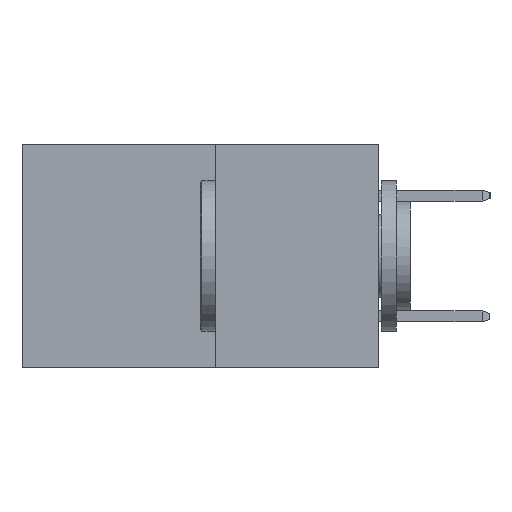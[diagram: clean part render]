
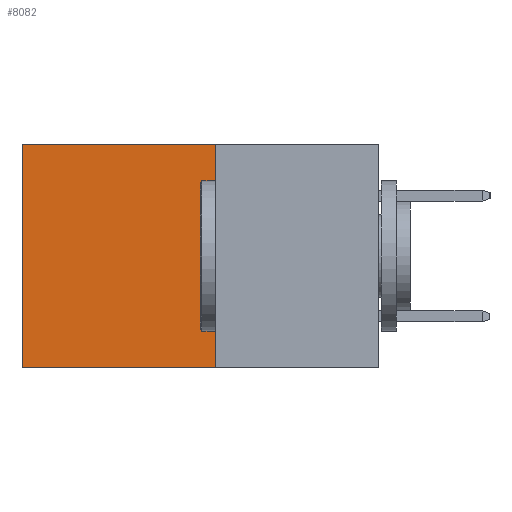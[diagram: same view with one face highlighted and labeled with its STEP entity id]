
A CAD part, left-side view. The second image highlights one B-rep face of the part: STEP entity #8082.
In plain terms, the highlighted planar face has unit normal (-1, 0, 0).
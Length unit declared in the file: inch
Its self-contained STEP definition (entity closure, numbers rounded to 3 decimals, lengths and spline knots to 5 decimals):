
#950 = CARTESIAN_POINT ( 'NONE',  ( 0.277, 0.27, -0.37 ) ) ;
#1495 = DIRECTION ( 'NONE',  ( 0., 0., -1. ) ) ;
#1499 = DIRECTION ( 'NONE',  ( 1., 0., 0. ) ) ;
#1833 = PLANE ( 'NONE',  #4125 ) ;
#2348 = EDGE_CURVE ( 'NONE', #11080, #16484, #6023, .T. ) ;
#2470 = VECTOR ( 'NONE', #13514, 39.37008 ) ;
#2774 = CARTESIAN_POINT ( 'NONE',  ( 0.277, 0.59, -0.37 ) ) ;
#3952 = CARTESIAN_POINT ( 'NONE',  ( 0.277, 0.27, -0.37 ) ) ;
#4125 = AXIS2_PLACEMENT_3D ( 'NONE', #950, #1499, #1495 ) ;
#5285 = CARTESIAN_POINT ( 'NONE',  ( 0.277, 0.27, -0.37 ) ) ;
#5861 = DIRECTION ( 'NONE',  ( 0., 0., -1. ) ) ;
#6023 = LINE ( 'NONE', #19803, #14229 ) ;
#6174 = ORIENTED_EDGE ( 'NONE', *, *, #2348, .T. ) ;
#6999 = CARTESIAN_POINT ( 'NONE',  ( 0.277, 0.27, 0. ) ) ;
#7414 = CARTESIAN_POINT ( 'NONE',  ( 0.277, 0.59, -0.37 ) ) ;
#8048 = VERTEX_POINT ( 'NONE', #2774 ) ;
#8082 = ADVANCED_FACE ( 'NONE', ( #18845 ), #1833, .F. ) ;
#9670 = ORIENTED_EDGE ( 'NONE', *, *, #15406, .T. ) ;
#11046 = EDGE_CURVE ( 'NONE', #13710, #8048, #16786, .T. ) ;
#11080 = VERTEX_POINT ( 'NONE', #6999 ) ;
#11224 = LINE ( 'NONE', #5285, #2470 ) ;
#11816 = CARTESIAN_POINT ( 'NONE',  ( 0.277, 0.27, -0.37 ) ) ;
#13383 = CARTESIAN_POINT ( 'NONE',  ( 0.277, 0.59, 0. ) ) ;
#13514 = DIRECTION ( 'NONE',  ( 0., 0., -1. ) ) ;
#13710 = VERTEX_POINT ( 'NONE', #3952 ) ;
#14229 = VECTOR ( 'NONE', #18562, 39.37008 ) ;
#15125 = DIRECTION ( 'NONE',  ( 0., 1., 0. ) ) ;
#15187 = EDGE_CURVE ( 'NONE', #11080, #13710, #11224, .T. ) ;
#15406 = EDGE_CURVE ( 'NONE', #16484, #8048, #19935, .T. ) ;
#15818 = VECTOR ( 'NONE', #15125, 39.37008 ) ;
#15825 = VECTOR ( 'NONE', #5861, 39.37008 ) ;
#16484 = VERTEX_POINT ( 'NONE', #13383 ) ;
#16786 = LINE ( 'NONE', #11816, #15818 ) ;
#17423 = ORIENTED_EDGE ( 'NONE', *, *, #15187, .F. ) ;
#17851 = EDGE_LOOP ( 'NONE', ( #9670, #19090, #17423, #6174 ) ) ;
#18562 = DIRECTION ( 'NONE',  ( 0., 1., 0. ) ) ;
#18845 = FACE_OUTER_BOUND ( 'NONE', #17851, .T. ) ;
#19090 = ORIENTED_EDGE ( 'NONE', *, *, #11046, .F. ) ;
#19803 = CARTESIAN_POINT ( 'NONE',  ( 0.277, 0.27, 0. ) ) ;
#19935 = LINE ( 'NONE', #7414, #15825 ) ;
